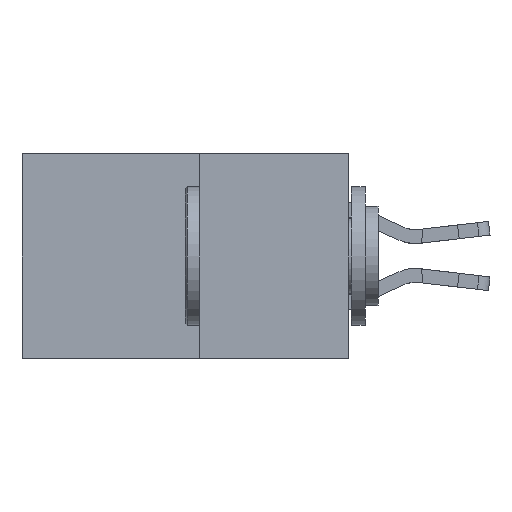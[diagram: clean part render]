
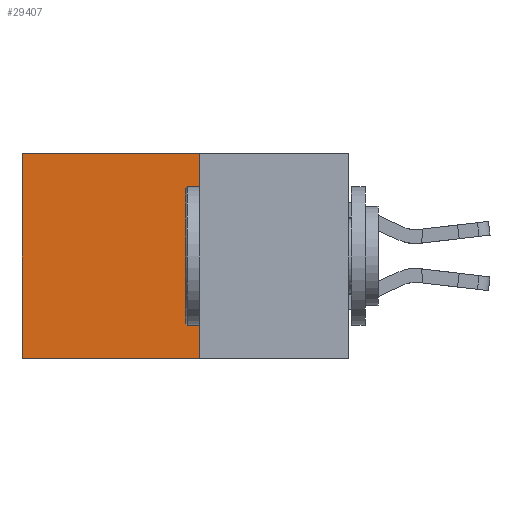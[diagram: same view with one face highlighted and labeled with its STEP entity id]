
A CAD part, left-side view. The second image highlights one B-rep face of the part: STEP entity #29407.
In plain terms, the highlighted planar face has unit normal (-1, 0, 0).
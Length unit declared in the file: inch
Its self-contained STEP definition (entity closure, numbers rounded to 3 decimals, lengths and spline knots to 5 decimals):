
#256 = ORIENTED_EDGE ( 'NONE', *, *, #25759, .F. ) ;
#468 = CARTESIAN_POINT ( 'NONE',  ( 0.277, 0.27, 0. ) ) ;
#643 = VERTEX_POINT ( 'NONE', #26238 ) ;
#3644 = VERTEX_POINT ( 'NONE', #29019 ) ;
#3795 = VECTOR ( 'NONE', #15030, 39.37008 ) ;
#4459 = CARTESIAN_POINT ( 'NONE',  ( 0.277, 0.59, -0.37 ) ) ;
#4688 = CARTESIAN_POINT ( 'NONE',  ( 0.277, 0.27, -0.37 ) ) ;
#6231 = FACE_OUTER_BOUND ( 'NONE', #27637, .T. ) ;
#8529 = CARTESIAN_POINT ( 'NONE',  ( 0.277, 0.59, -0.37 ) ) ;
#8659 = EDGE_CURVE ( 'NONE', #3644, #16756, #12875, .T. ) ;
#9854 = EDGE_CURVE ( 'NONE', #643, #16756, #24438, .T. ) ;
#10185 = VECTOR ( 'NONE', #14502, 39.37008 ) ;
#10691 = AXIS2_PLACEMENT_3D ( 'NONE', #21015, #13878, #30419 ) ;
#12016 = CARTESIAN_POINT ( 'NONE',  ( 0.277, 0.27, -0.37 ) ) ;
#12875 = LINE ( 'NONE', #12016, #10185 ) ;
#13878 = DIRECTION ( 'NONE',  ( 1., 0., 0. ) ) ;
#14327 = DIRECTION ( 'NONE',  ( 0., 0., -1. ) ) ;
#14502 = DIRECTION ( 'NONE',  ( 0., 1., 0. ) ) ;
#15030 = DIRECTION ( 'NONE',  ( 0., 1., 0. ) ) ;
#16756 = VERTEX_POINT ( 'NONE', #4459 ) ;
#18117 = ORIENTED_EDGE ( 'NONE', *, *, #8659, .F. ) ;
#18142 = VECTOR ( 'NONE', #30018, 39.37008 ) ;
#18883 = VERTEX_POINT ( 'NONE', #25713 ) ;
#19009 = VECTOR ( 'NONE', #14327, 39.37008 ) ;
#19609 = ORIENTED_EDGE ( 'NONE', *, *, #29722, .T. ) ;
#21015 = CARTESIAN_POINT ( 'NONE',  ( 0.277, 0.27, -0.37 ) ) ;
#22298 = LINE ( 'NONE', #468, #3795 ) ;
#24438 = LINE ( 'NONE', #8529, #18142 ) ;
#25316 = LINE ( 'NONE', #4688, #19009 ) ;
#25713 = CARTESIAN_POINT ( 'NONE',  ( 0.277, 0.27, 0. ) ) ;
#25759 = EDGE_CURVE ( 'NONE', #18883, #3644, #25316, .T. ) ;
#26238 = CARTESIAN_POINT ( 'NONE',  ( 0.277, 0.59, 0. ) ) ;
#26300 = ORIENTED_EDGE ( 'NONE', *, *, #9854, .T. ) ;
#27637 = EDGE_LOOP ( 'NONE', ( #26300, #18117, #256, #19609 ) ) ;
#28107 = PLANE ( 'NONE',  #10691 ) ;
#29019 = CARTESIAN_POINT ( 'NONE',  ( 0.277, 0.27, -0.37 ) ) ;
#29407 = ADVANCED_FACE ( 'NONE', ( #6231 ), #28107, .F. ) ;
#29722 = EDGE_CURVE ( 'NONE', #18883, #643, #22298, .T. ) ;
#30018 = DIRECTION ( 'NONE',  ( 0., 0., -1. ) ) ;
#30419 = DIRECTION ( 'NONE',  ( 0., 0., -1. ) ) ;
